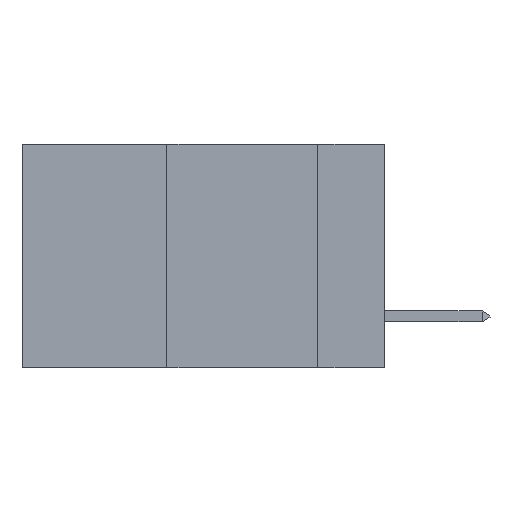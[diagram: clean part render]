
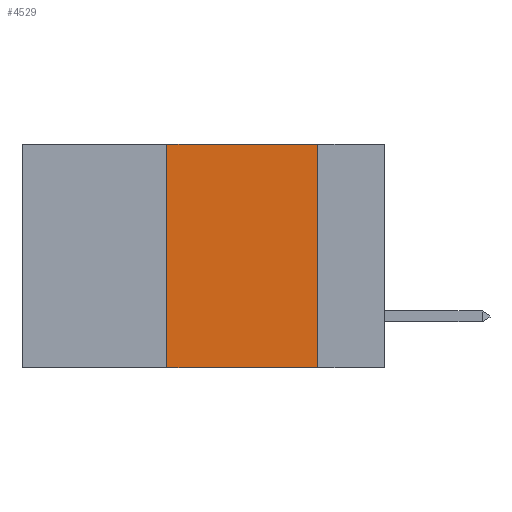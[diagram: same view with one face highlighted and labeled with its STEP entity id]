
A CAD part, left-side view. The second image highlights one B-rep face of the part: STEP entity #4529.
In plain terms, the highlighted planar face has unit normal (-1, 0, 0).
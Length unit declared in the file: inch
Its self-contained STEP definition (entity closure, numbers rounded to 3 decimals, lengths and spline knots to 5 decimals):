
#1615 = VERTEX_POINT ( 'NONE', #28389 ) ;
#1677 = EDGE_LOOP ( 'NONE', ( #6071, #23079, #29005, #17870 ) ) ;
#2231 = PLANE ( 'NONE',  #3696 ) ;
#2371 = VECTOR ( 'NONE', #21401, 39.37008 ) ;
#2525 = CARTESIAN_POINT ( 'NONE',  ( 0., 0.6, 0. ) ) ;
#2590 = LINE ( 'NONE', #8912, #20703 ) ;
#3110 = LINE ( 'NONE', #2525, #2371 ) ;
#3696 = AXIS2_PLACEMENT_3D ( 'NONE', #30250, #4589, #21117 ) ;
#4529 = ADVANCED_FACE ( 'NONE', ( #22116 ), #2231, .F. ) ;
#4589 = DIRECTION ( 'NONE',  ( 1., 0., 0. ) ) ;
#6071 = ORIENTED_EDGE ( 'NONE', *, *, #8312, .F. ) ;
#6877 = CARTESIAN_POINT ( 'NONE',  ( 0., 0.36, -0.37 ) ) ;
#8312 = EDGE_CURVE ( 'NONE', #21700, #10491, #26630, .T. ) ;
#8912 = CARTESIAN_POINT ( 'NONE',  ( 0., 0.6, -0.37 ) ) ;
#9561 = CARTESIAN_POINT ( 'NONE',  ( 0., 0.11, 0. ) ) ;
#10491 = VERTEX_POINT ( 'NONE', #19969 ) ;
#12238 = VERTEX_POINT ( 'NONE', #6877 ) ;
#14714 = EDGE_CURVE ( 'NONE', #12238, #1615, #27648, .T. ) ;
#14773 = CARTESIAN_POINT ( 'NONE',  ( 0., 0.11, 0. ) ) ;
#14985 = VECTOR ( 'NONE', #28366, 39.37008 ) ;
#15231 = VECTOR ( 'NONE', #18375, 39.37008 ) ;
#16005 = CARTESIAN_POINT ( 'NONE',  ( 0., 0.36, 0. ) ) ;
#17870 = ORIENTED_EDGE ( 'NONE', *, *, #19409, .T. ) ;
#18375 = DIRECTION ( 'NONE',  ( 0., 0., 1. ) ) ;
#19409 = EDGE_CURVE ( 'NONE', #12238, #10491, #2590, .T. ) ;
#19969 = CARTESIAN_POINT ( 'NONE',  ( 0., 0.11, -0.37 ) ) ;
#20703 = VECTOR ( 'NONE', #25332, 39.37008 ) ;
#21117 = DIRECTION ( 'NONE',  ( 0., 0., -1. ) ) ;
#21401 = DIRECTION ( 'NONE',  ( 0., -1., 0. ) ) ;
#21700 = VERTEX_POINT ( 'NONE', #14773 ) ;
#22116 = FACE_OUTER_BOUND ( 'NONE', #1677, .T. ) ;
#22782 = EDGE_CURVE ( 'NONE', #1615, #21700, #3110, .T. ) ;
#23079 = ORIENTED_EDGE ( 'NONE', *, *, #22782, .F. ) ;
#25332 = DIRECTION ( 'NONE',  ( 0., -1., 0. ) ) ;
#26630 = LINE ( 'NONE', #9561, #14985 ) ;
#27648 = LINE ( 'NONE', #16005, #15231 ) ;
#28366 = DIRECTION ( 'NONE',  ( 0., 0., -1. ) ) ;
#28389 = CARTESIAN_POINT ( 'NONE',  ( 0., 0.36, 0. ) ) ;
#29005 = ORIENTED_EDGE ( 'NONE', *, *, #14714, .F. ) ;
#30250 = CARTESIAN_POINT ( 'NONE',  ( 0., 0.6, 0. ) ) ;
